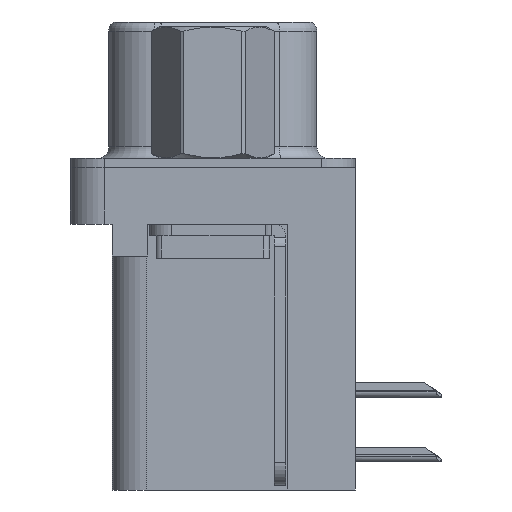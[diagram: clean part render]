
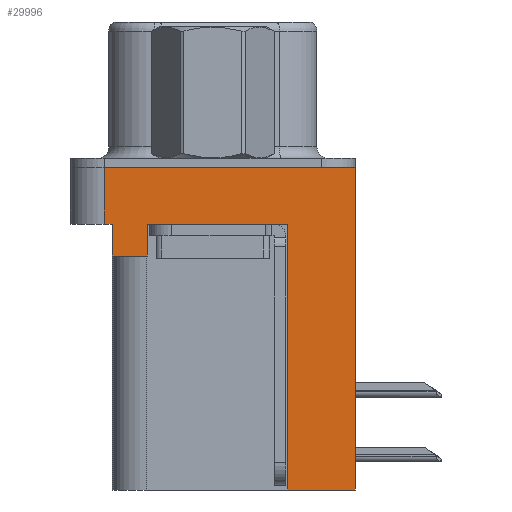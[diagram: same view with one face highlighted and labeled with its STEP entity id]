
A CAD part, left-side view. The second image highlights one B-rep face of the part: STEP entity #29996.
In plain terms, the highlighted planar face has unit normal (-1, 0, 0).
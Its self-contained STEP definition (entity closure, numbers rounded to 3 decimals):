
#83 = VECTOR ( 'NONE', #18441, 1000. ) ;
#720 = EDGE_CURVE ( 'NONE', #16480, #30250, #6066, .T. ) ;
#1162 = DIRECTION ( 'NONE',  ( 0., 0., 1. ) ) ;
#1180 = EDGE_CURVE ( 'NONE', #5322, #13110, #18451, .T. ) ;
#1204 = CARTESIAN_POINT ( 'NONE',  ( -2.91, 2.895, -3.9 ) ) ;
#1213 = CARTESIAN_POINT ( 'NONE',  ( -2.91, -6.275, -2.5 ) ) ;
#1312 = VERTEX_POINT ( 'NONE', #13352 ) ;
#1403 = CARTESIAN_POINT ( 'NONE',  ( -2.91, 2.895, -3.9 ) ) ;
#1487 = CARTESIAN_POINT ( 'NONE',  ( -2.91, -6.275, -2.5 ) ) ;
#1670 = CARTESIAN_POINT ( 'NONE',  ( -2.91, 4.425, -3.9 ) ) ;
#1834 = FACE_OUTER_BOUND ( 'NONE', #8051, .T. ) ;
#3062 = VECTOR ( 'NONE', #1162, 1000. ) ;
#3237 = EDGE_CURVE ( 'NONE', #31373, #13110, #8869, .T. ) ;
#3946 = VECTOR ( 'NONE', #15658, 1000. ) ;
#5322 = VERTEX_POINT ( 'NONE', #30166 ) ;
#5852 = EDGE_CURVE ( 'NONE', #17077, #19737, #22753, .T. ) ;
#6066 = LINE ( 'NONE', #1403, #3946 ) ;
#6382 = ORIENTED_EDGE ( 'NONE', *, *, #20935, .F. ) ;
#7013 = VECTOR ( 'NONE', #29950, 1000. ) ;
#7801 = EDGE_CURVE ( 'NONE', #30250, #19737, #21422, .T. ) ;
#7961 = VECTOR ( 'NONE', #14080, 1000. ) ;
#8051 = EDGE_LOOP ( 'NONE', ( #16649, #17035, #30885, #6382, #8201, #21927, #11900, #9228, #28811, #26026 ) ) ;
#8201 = ORIENTED_EDGE ( 'NONE', *, *, #15233, .F. ) ;
#8869 = LINE ( 'NONE', #1487, #3062 ) ;
#9228 = ORIENTED_EDGE ( 'NONE', *, *, #5852, .F. ) ;
#10054 = VECTOR ( 'NONE', #16246, 1000. ) ;
#10960 = CARTESIAN_POINT ( 'NONE',  ( -2.91, -6.275, 0. ) ) ;
#11900 = ORIENTED_EDGE ( 'NONE', *, *, #7801, .T. ) ;
#11951 = CARTESIAN_POINT ( 'NONE',  ( -2.91, -3.295, -2.5 ) ) ;
#13110 = VERTEX_POINT ( 'NONE', #23901 ) ;
#13352 = CARTESIAN_POINT ( 'NONE',  ( -2.91, 4.425, -2.5 ) ) ;
#13995 = PLANE ( 'NONE',  #25040 ) ;
#14080 = DIRECTION ( 'NONE',  ( 0., -1., 0. ) ) ;
#14174 = LINE ( 'NONE', #23907, #10054 ) ;
#15204 = LINE ( 'NONE', #24944, #29463 ) ;
#15233 = EDGE_CURVE ( 'NONE', #16480, #30080, #16681, .T. ) ;
#15658 = DIRECTION ( 'NONE',  ( 0., 0., 1. ) ) ;
#15917 = DIRECTION ( 'NONE',  ( -1., 0., 0. ) ) ;
#16246 = DIRECTION ( 'NONE',  ( 0., 1., 0. ) ) ;
#16480 = VERTEX_POINT ( 'NONE', #1204 ) ;
#16563 = VECTOR ( 'NONE', #24159, 1000. ) ;
#16649 = ORIENTED_EDGE ( 'NONE', *, *, #1180, .F. ) ;
#16681 = LINE ( 'NONE', #26431, #83 ) ;
#17035 = ORIENTED_EDGE ( 'NONE', *, *, #23376, .F. ) ;
#17077 = VERTEX_POINT ( 'NONE', #26527 ) ;
#17393 = EDGE_CURVE ( 'NONE', #18309, #1312, #25850, .T. ) ;
#18000 = CARTESIAN_POINT ( 'NONE',  ( -2.91, 4.775, -2.5 ) ) ;
#18307 = CARTESIAN_POINT ( 'NONE',  ( -2.91, -6.275, -2.5 ) ) ;
#18309 = VERTEX_POINT ( 'NONE', #18000 ) ;
#18441 = DIRECTION ( 'NONE',  ( 0., 1., 0. ) ) ;
#18451 = LINE ( 'NONE', #10960, #27464 ) ;
#18899 = LINE ( 'NONE', #28973, #16563 ) ;
#19737 = VERTEX_POINT ( 'NONE', #11951 ) ;
#20042 = CARTESIAN_POINT ( 'NONE',  ( -2.91, -3.295, -14.2 ) ) ;
#20935 = EDGE_CURVE ( 'NONE', #30080, #1312, #18899, .T. ) ;
#21422 = LINE ( 'NONE', #26224, #7961 ) ;
#21819 = CARTESIAN_POINT ( 'NONE',  ( -2.91, 2.895, -2.5 ) ) ;
#21927 = ORIENTED_EDGE ( 'NONE', *, *, #720, .T. ) ;
#22378 = EDGE_CURVE ( 'NONE', #31373, #17077, #14174, .T. ) ;
#22753 = LINE ( 'NONE', #20042, #7013 ) ;
#22949 = CARTESIAN_POINT ( 'NONE',  ( -2.91, -6.275, -14.2 ) ) ;
#23376 = EDGE_CURVE ( 'NONE', #18309, #5322, #15204, .T. ) ;
#23901 = CARTESIAN_POINT ( 'NONE',  ( -2.91, -6.275, 0. ) ) ;
#23907 = CARTESIAN_POINT ( 'NONE',  ( -2.91, -3.295, -14.2 ) ) ;
#24159 = DIRECTION ( 'NONE',  ( 0., 0., 1. ) ) ;
#24944 = CARTESIAN_POINT ( 'NONE',  ( -2.91, 4.775, -2.5 ) ) ;
#25040 = AXIS2_PLACEMENT_3D ( 'NONE', #18307, #15917, #30782 ) ;
#25091 = DIRECTION ( 'NONE',  ( 0., 0., 1. ) ) ;
#25530 = DIRECTION ( 'NONE',  ( 0., -1., 0. ) ) ;
#25850 = LINE ( 'NONE', #1213, #28780 ) ;
#26026 = ORIENTED_EDGE ( 'NONE', *, *, #3237, .T. ) ;
#26124 = DIRECTION ( 'NONE',  ( 0., -1., 0. ) ) ;
#26224 = CARTESIAN_POINT ( 'NONE',  ( -2.91, -6.275, -2.5 ) ) ;
#26431 = CARTESIAN_POINT ( 'NONE',  ( -2.91, 4.425, -3.9 ) ) ;
#26527 = CARTESIAN_POINT ( 'NONE',  ( -2.91, -3.295, -14.2 ) ) ;
#27464 = VECTOR ( 'NONE', #26124, 1000. ) ;
#28780 = VECTOR ( 'NONE', #25530, 1000. ) ;
#28811 = ORIENTED_EDGE ( 'NONE', *, *, #22378, .F. ) ;
#28973 = CARTESIAN_POINT ( 'NONE',  ( -2.91, 4.425, -3.9 ) ) ;
#29463 = VECTOR ( 'NONE', #25091, 1000. ) ;
#29950 = DIRECTION ( 'NONE',  ( 0., 0., 1. ) ) ;
#29996 = ADVANCED_FACE ( 'NONE', ( #1834 ), #13995, .T. ) ;
#30080 = VERTEX_POINT ( 'NONE', #1670 ) ;
#30166 = CARTESIAN_POINT ( 'NONE',  ( -2.91, 4.775, 0. ) ) ;
#30250 = VERTEX_POINT ( 'NONE', #21819 ) ;
#30782 = DIRECTION ( 'NONE',  ( 0., 0., 1. ) ) ;
#30885 = ORIENTED_EDGE ( 'NONE', *, *, #17393, .T. ) ;
#31373 = VERTEX_POINT ( 'NONE', #22949 ) ;
